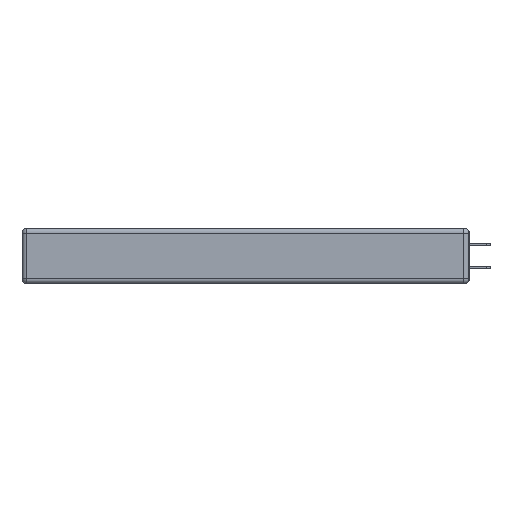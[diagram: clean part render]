
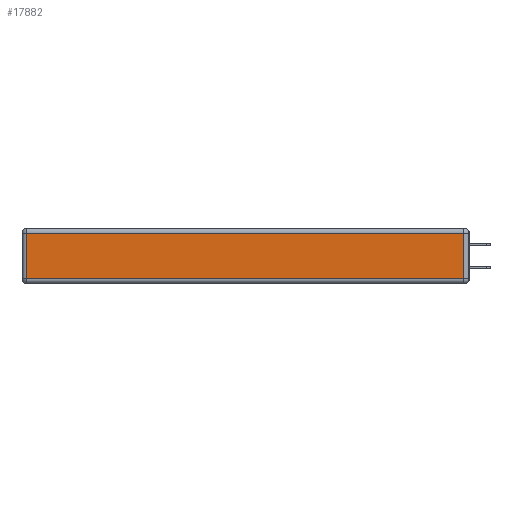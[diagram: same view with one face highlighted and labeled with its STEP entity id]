
A CAD part, left-side view. The second image highlights one B-rep face of the part: STEP entity #17882.
In plain terms, the highlighted planar face has unit normal (-1, 0, 0).
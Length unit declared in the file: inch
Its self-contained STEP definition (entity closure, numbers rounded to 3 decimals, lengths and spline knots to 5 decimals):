
#688 = DIRECTION ( 'NONE',  ( 0., 1., 0. ) ) ;
#705 = EDGE_CURVE ( 'NONE', #13168, #13381, #24560, .T. ) ;
#1057 = LINE ( 'NONE', #19636, #3749 ) ;
#1217 = ORIENTED_EDGE ( 'NONE', *, *, #705, .T. ) ;
#1274 = LINE ( 'NONE', #20708, #19673 ) ;
#3749 = VECTOR ( 'NONE', #9848, 39.37008 ) ;
#4492 = DIRECTION ( 'NONE',  ( 0., 0., 1. ) ) ;
#5089 = EDGE_CURVE ( 'NONE', #13381, #20763, #1274, .T. ) ;
#5204 = CARTESIAN_POINT ( 'NONE',  ( 0., 2.72, -0.313 ) ) ;
#6598 = CARTESIAN_POINT ( 'NONE',  ( 0., 0.03, -0.313 ) ) ;
#9848 = DIRECTION ( 'NONE',  ( 0., 0., -1. ) ) ;
#10379 = DIRECTION ( 'NONE',  ( 0., -1., 0. ) ) ;
#13168 = VERTEX_POINT ( 'NONE', #6598 ) ;
#13381 = VERTEX_POINT ( 'NONE', #14459 ) ;
#14459 = CARTESIAN_POINT ( 'NONE',  ( 0., 0.03, -0.03 ) ) ;
#15423 = DIRECTION ( 'NONE',  ( -1., 0., 0. ) ) ;
#15810 = EDGE_CURVE ( 'NONE', #19291, #13168, #30734, .T. ) ;
#17882 = ADVANCED_FACE ( 'NONE', ( #26869 ), #24798, .T. ) ;
#17947 = ORIENTED_EDGE ( 'NONE', *, *, #15810, .T. ) ;
#17995 = CARTESIAN_POINT ( 'NONE',  ( 0., 0., -0.343 ) ) ;
#18756 = VECTOR ( 'NONE', #4492, 39.37008 ) ;
#19157 = CARTESIAN_POINT ( 'NONE',  ( 0., 0.03, -0.343 ) ) ;
#19291 = VERTEX_POINT ( 'NONE', #5204 ) ;
#19624 = ORIENTED_EDGE ( 'NONE', *, *, #5089, .T. ) ;
#19636 = CARTESIAN_POINT ( 'NONE',  ( 0., 2.72, -0.343 ) ) ;
#19673 = VECTOR ( 'NONE', #688, 39.37008 ) ;
#20708 = CARTESIAN_POINT ( 'NONE',  ( 0., 2.75, -0.03 ) ) ;
#20763 = VERTEX_POINT ( 'NONE', #27958 ) ;
#21335 = AXIS2_PLACEMENT_3D ( 'NONE', #17995, #15423, #23087 ) ;
#22669 = CARTESIAN_POINT ( 'NONE',  ( 0., 0., -0.313 ) ) ;
#23087 = DIRECTION ( 'NONE',  ( 0., 0., 1. ) ) ;
#24223 = VECTOR ( 'NONE', #10379, 39.37008 ) ;
#24560 = LINE ( 'NONE', #19157, #18756 ) ;
#24798 = PLANE ( 'NONE',  #21335 ) ;
#26869 = FACE_OUTER_BOUND ( 'NONE', #29787, .T. ) ;
#27958 = CARTESIAN_POINT ( 'NONE',  ( 0., 2.72, -0.03 ) ) ;
#29787 = EDGE_LOOP ( 'NONE', ( #17947, #1217, #19624, #31220 ) ) ;
#30734 = LINE ( 'NONE', #22669, #24223 ) ;
#31220 = ORIENTED_EDGE ( 'NONE', *, *, #31383, .T. ) ;
#31383 = EDGE_CURVE ( 'NONE', #20763, #19291, #1057, .T. ) ;
